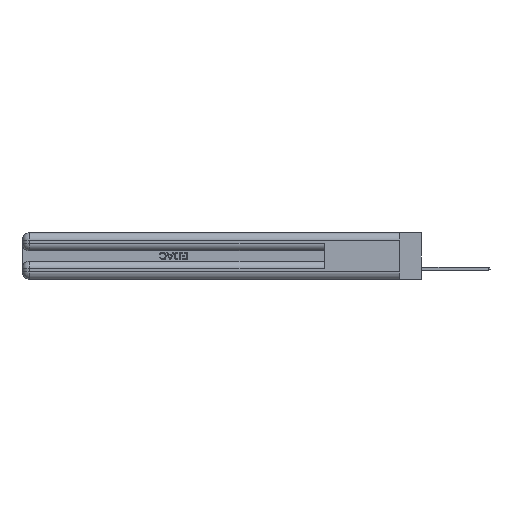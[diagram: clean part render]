
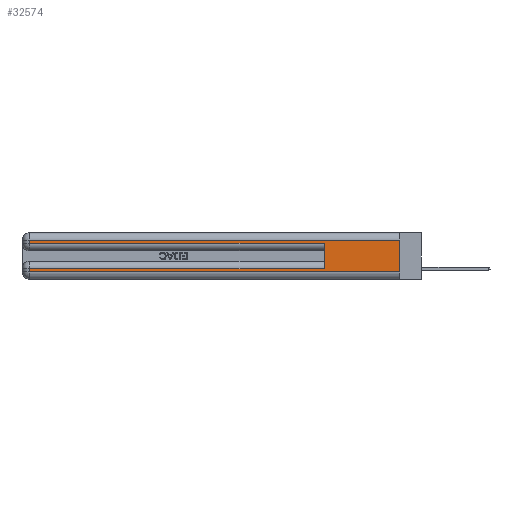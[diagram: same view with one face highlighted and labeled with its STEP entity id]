
A CAD part, left-side view. The second image highlights one B-rep face of the part: STEP entity #32574.
In plain terms, the highlighted planar face has unit normal (-1, 0, 0).
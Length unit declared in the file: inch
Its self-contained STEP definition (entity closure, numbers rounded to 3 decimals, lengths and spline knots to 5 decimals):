
#433 = VECTOR ( 'NONE', #38403, 39.37008 ) ;
#1590 = CARTESIAN_POINT ( 'NONE',  ( 0., 0., 0.31 ) ) ;
#2196 = CARTESIAN_POINT ( 'NONE',  ( 0., 0.6, 0.285 ) ) ;
#5113 = LINE ( 'NONE', #34682, #433 ) ;
#5213 = VERTEX_POINT ( 'NONE', #13754 ) ;
#5287 = EDGE_CURVE ( 'NONE', #29702, #47570, #26880, .T. ) ;
#6129 = DIRECTION ( 'NONE',  ( 0., 0., -1. ) ) ;
#7492 = CARTESIAN_POINT ( 'NONE',  ( 0., 2.94, 0.085 ) ) ;
#8590 = DIRECTION ( 'NONE',  ( 0., 1., 0. ) ) ;
#9726 = EDGE_CURVE ( 'NONE', #38410, #33676, #18931, .T. ) ;
#9991 = VECTOR ( 'NONE', #26631, 39.37008 ) ;
#10331 = ORIENTED_EDGE ( 'NONE', *, *, #26361, .T. ) ;
#10547 = DIRECTION ( 'NONE',  ( 0., -1., 0. ) ) ;
#10801 = LINE ( 'NONE', #43259, #45497 ) ;
#13754 = CARTESIAN_POINT ( 'NONE',  ( 0., 2.94, 0.285 ) ) ;
#15372 = CARTESIAN_POINT ( 'NONE',  ( 0., 2.94, 0.06 ) ) ;
#16008 = CARTESIAN_POINT ( 'NONE',  ( 0., 0., 0.085 ) ) ;
#16817 = EDGE_CURVE ( 'NONE', #18544, #21072, #10801, .T. ) ;
#17124 = CARTESIAN_POINT ( 'NONE',  ( 0., 2.94, 0.37 ) ) ;
#17473 = LINE ( 'NONE', #44740, #9991 ) ;
#18544 = VERTEX_POINT ( 'NONE', #36908 ) ;
#18931 = LINE ( 'NONE', #1590, #36370 ) ;
#20116 = EDGE_CURVE ( 'NONE', #21605, #29702, #34777, .T. ) ;
#20343 = EDGE_CURVE ( 'NONE', #38410, #47570, #5113, .T. ) ;
#20636 = ORIENTED_EDGE ( 'NONE', *, *, #5287, .T. ) ;
#21072 = VERTEX_POINT ( 'NONE', #2196 ) ;
#21348 = VECTOR ( 'NONE', #28020, 39.37008 ) ;
#21605 = VERTEX_POINT ( 'NONE', #7492 ) ;
#21661 = VECTOR ( 'NONE', #10547, 39.37008 ) ;
#22085 = ORIENTED_EDGE ( 'NONE', *, *, #30049, .T. ) ;
#24858 = LINE ( 'NONE', #42113, #21348 ) ;
#26361 = EDGE_CURVE ( 'NONE', #18544, #21605, #29110, .T. ) ;
#26631 = DIRECTION ( 'NONE',  ( 0., 0., -1. ) ) ;
#26677 = ORIENTED_EDGE ( 'NONE', *, *, #16817, .F. ) ;
#26880 = LINE ( 'NONE', #39709, #21661 ) ;
#27590 = DIRECTION ( 'NONE',  ( 0., 1., 0. ) ) ;
#28020 = DIRECTION ( 'NONE',  ( 0., -1., 0. ) ) ;
#28066 = DIRECTION ( 'NONE',  ( 0., 0., 1. ) ) ;
#28372 = EDGE_LOOP ( 'NONE', ( #37027, #29720, #47941, #22085, #26677, #10331, #42539, #20636 ) ) ;
#29110 = LINE ( 'NONE', #16008, #32576 ) ;
#29702 = VERTEX_POINT ( 'NONE', #15372 ) ;
#29720 = ORIENTED_EDGE ( 'NONE', *, *, #9726, .T. ) ;
#29936 = CARTESIAN_POINT ( 'NONE',  ( 0., 2.94, 0.31 ) ) ;
#30049 = EDGE_CURVE ( 'NONE', #5213, #21072, #24858, .T. ) ;
#32574 = ADVANCED_FACE ( 'NONE', ( #46569 ), #34718, .F. ) ;
#32576 = VECTOR ( 'NONE', #8590, 39.37008 ) ;
#33676 = VERTEX_POINT ( 'NONE', #29936 ) ;
#34550 = CARTESIAN_POINT ( 'NONE',  ( 0., 0., 0.06 ) ) ;
#34682 = CARTESIAN_POINT ( 'NONE',  ( 0., 0., 0.37 ) ) ;
#34718 = PLANE ( 'NONE',  #37029 ) ;
#34777 = LINE ( 'NONE', #17124, #46287 ) ;
#36370 = VECTOR ( 'NONE', #27590, 39.37008 ) ;
#36908 = CARTESIAN_POINT ( 'NONE',  ( 0., 0.6, 0.085 ) ) ;
#37027 = ORIENTED_EDGE ( 'NONE', *, *, #20343, .F. ) ;
#37029 = AXIS2_PLACEMENT_3D ( 'NONE', #38280, #41681, #45672 ) ;
#38280 = CARTESIAN_POINT ( 'NONE',  ( 0., 0., 0.37 ) ) ;
#38403 = DIRECTION ( 'NONE',  ( 0., 0., -1. ) ) ;
#38410 = VERTEX_POINT ( 'NONE', #40677 ) ;
#39709 = CARTESIAN_POINT ( 'NONE',  ( 0., 0., 0.06 ) ) ;
#40677 = CARTESIAN_POINT ( 'NONE',  ( 0., 0., 0.31 ) ) ;
#41681 = DIRECTION ( 'NONE',  ( 1., 0., 0. ) ) ;
#42113 = CARTESIAN_POINT ( 'NONE',  ( 0., 0., 0.285 ) ) ;
#42539 = ORIENTED_EDGE ( 'NONE', *, *, #20116, .T. ) ;
#43259 = CARTESIAN_POINT ( 'NONE',  ( 0., 0.6, 0.145 ) ) ;
#44194 = EDGE_CURVE ( 'NONE', #33676, #5213, #17473, .T. ) ;
#44740 = CARTESIAN_POINT ( 'NONE',  ( 0., 2.94, 0.37 ) ) ;
#45497 = VECTOR ( 'NONE', #28066, 39.37008 ) ;
#45672 = DIRECTION ( 'NONE',  ( 0., 0., -1. ) ) ;
#46287 = VECTOR ( 'NONE', #6129, 39.37008 ) ;
#46569 = FACE_OUTER_BOUND ( 'NONE', #28372, .T. ) ;
#47570 = VERTEX_POINT ( 'NONE', #34550 ) ;
#47941 = ORIENTED_EDGE ( 'NONE', *, *, #44194, .T. ) ;
